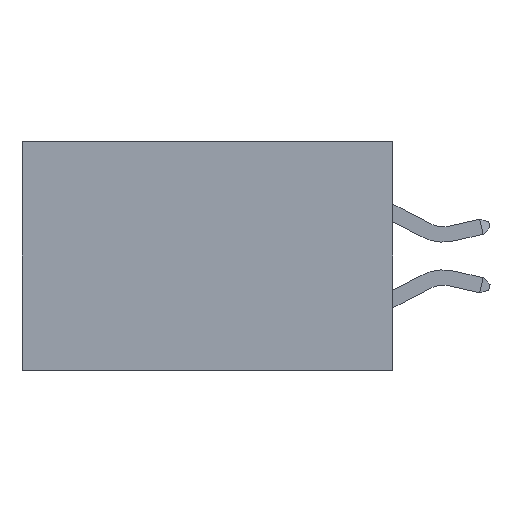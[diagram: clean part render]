
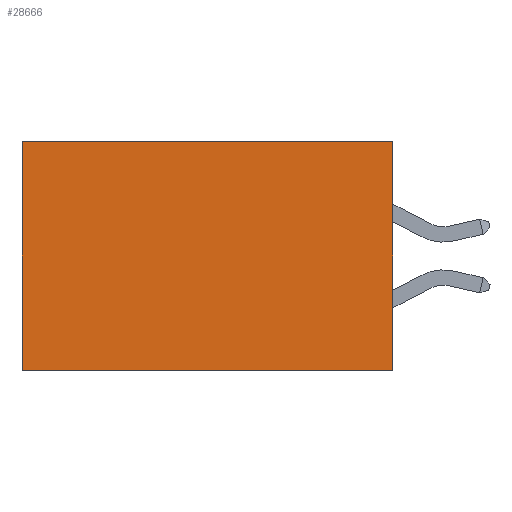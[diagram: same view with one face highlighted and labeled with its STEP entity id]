
A CAD part, left-side view. The second image highlights one B-rep face of the part: STEP entity #28666.
In plain terms, the highlighted planar face has unit normal (-1, 0, 0).
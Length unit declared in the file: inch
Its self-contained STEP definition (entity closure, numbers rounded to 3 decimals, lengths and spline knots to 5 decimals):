
#567 = ORIENTED_EDGE ( 'NONE', *, *, #22333, .F. ) ;
#916 = LINE ( 'NONE', #13385, #5549 ) ;
#1225 = EDGE_CURVE ( 'NONE', #10471, #5928, #24102, .T. ) ;
#3047 = CARTESIAN_POINT ( 'NONE',  ( 0.2875, 0., -0.37 ) ) ;
#4246 = ORIENTED_EDGE ( 'NONE', *, *, #1225, .T. ) ;
#4627 = VECTOR ( 'NONE', #19228, 39.37008 ) ;
#5173 = CARTESIAN_POINT ( 'NONE',  ( 0.2875, 0., 0. ) ) ;
#5258 = CARTESIAN_POINT ( 'NONE',  ( 0.2875, 0.6, -0.37 ) ) ;
#5463 = DIRECTION ( 'NONE',  ( 0., 1., 0. ) ) ;
#5549 = VECTOR ( 'NONE', #22789, 39.37008 ) ;
#5928 = VERTEX_POINT ( 'NONE', #5258 ) ;
#7094 = LINE ( 'NONE', #3047, #23222 ) ;
#8924 = CARTESIAN_POINT ( 'NONE',  ( 0.2875, 0.6, 0. ) ) ;
#10471 = VERTEX_POINT ( 'NONE', #13097 ) ;
#11754 = ORIENTED_EDGE ( 'NONE', *, *, #16469, .T. ) ;
#13097 = CARTESIAN_POINT ( 'NONE',  ( 0.2875, 0.6, 0. ) ) ;
#13242 = LINE ( 'NONE', #23926, #4627 ) ;
#13385 = CARTESIAN_POINT ( 'NONE',  ( 0.2875, 0., 0. ) ) ;
#13619 = CARTESIAN_POINT ( 'NONE',  ( 0.2875, 0., -0.37 ) ) ;
#15448 = ORIENTED_EDGE ( 'NONE', *, *, #17055, .F. ) ;
#16469 = EDGE_CURVE ( 'NONE', #16959, #10471, #13242, .T. ) ;
#16959 = VERTEX_POINT ( 'NONE', #5173 ) ;
#17055 = EDGE_CURVE ( 'NONE', #27668, #5928, #7094, .T. ) ;
#17619 = PLANE ( 'NONE',  #28413 ) ;
#17918 = DIRECTION ( 'NONE',  ( 0., 0., -1. ) ) ;
#19047 = EDGE_LOOP ( 'NONE', ( #4246, #15448, #567, #11754 ) ) ;
#19228 = DIRECTION ( 'NONE',  ( 0., 1., 0. ) ) ;
#22172 = FACE_OUTER_BOUND ( 'NONE', #19047, .T. ) ;
#22216 = CARTESIAN_POINT ( 'NONE',  ( 0.2875, 0., 0. ) ) ;
#22323 = DIRECTION ( 'NONE',  ( 1., 0., 0. ) ) ;
#22333 = EDGE_CURVE ( 'NONE', #16959, #27668, #916, .T. ) ;
#22530 = DIRECTION ( 'NONE',  ( 0., 0., -1. ) ) ;
#22789 = DIRECTION ( 'NONE',  ( 0., 0., -1. ) ) ;
#23222 = VECTOR ( 'NONE', #5463, 39.37008 ) ;
#23398 = VECTOR ( 'NONE', #22530, 39.37008 ) ;
#23926 = CARTESIAN_POINT ( 'NONE',  ( 0.2875, 0., 0. ) ) ;
#24102 = LINE ( 'NONE', #8924, #23398 ) ;
#27668 = VERTEX_POINT ( 'NONE', #13619 ) ;
#28413 = AXIS2_PLACEMENT_3D ( 'NONE', #22216, #22323, #17918 ) ;
#28666 = ADVANCED_FACE ( 'NONE', ( #22172 ), #17619, .F. ) ;
